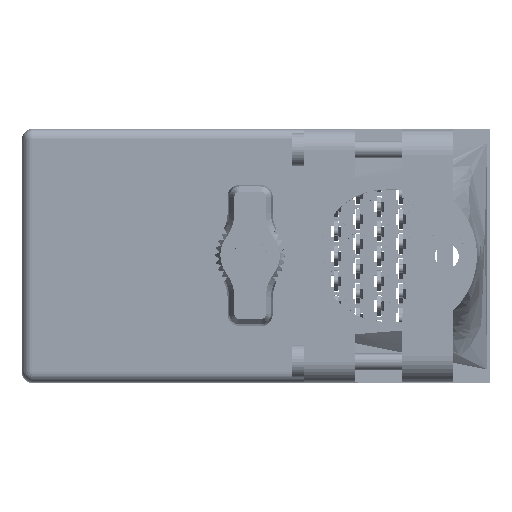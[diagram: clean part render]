
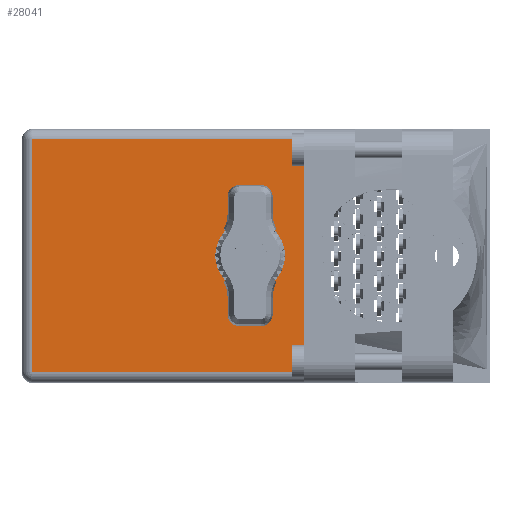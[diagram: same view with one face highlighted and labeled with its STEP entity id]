
A CAD part, top view. The second image highlights one B-rep face of the part: STEP entity #28041.
In plain terms, the highlighted face is planar.
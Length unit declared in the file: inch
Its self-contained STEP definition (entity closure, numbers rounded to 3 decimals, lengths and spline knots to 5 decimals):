
#1946 = DIRECTION ( 'NONE',  ( 1., 0., 0. ) ) ;
#2093 = VERTEX_POINT ( 'NONE', #85353 ) ;
#4004 = CARTESIAN_POINT ( 'NONE',  ( 1.3775, 2.03, -0.765 ) ) ;
#4161 = ORIENTED_EDGE ( 'NONE', *, *, #67292, .T. ) ;
#4527 = AXIS2_PLACEMENT_3D ( 'NONE', #5565, #39660, #73638 ) ;
#4906 = VECTOR ( 'NONE', #41495, 39.37008 ) ;
#5565 = CARTESIAN_POINT ( 'NONE',  ( 0., 2.03, -1.53 ) ) ;
#7499 = CARTESIAN_POINT ( 'NONE',  ( 1.3775, 2.03, -0.6635 ) ) ;
#7896 = CIRCLE ( 'NONE', #96307, 0.1015 ) ;
#8523 = DIRECTION ( 'NONE',  ( -1., 0., 0. ) ) ;
#12904 = VERTEX_POINT ( 'NONE', #34592 ) ;
#14718 = CARTESIAN_POINT ( 'NONE',  ( 1.705, 2.03, -1.468 ) ) ;
#15631 = VECTOR ( 'NONE', #1946, 39.37008 ) ;
#16654 = ORIENTED_EDGE ( 'NONE', *, *, #51481, .F. ) ;
#16913 = LINE ( 'NONE', #26001, #15631 ) ;
#18015 = FACE_OUTER_BOUND ( 'NONE', #84927, .T. ) ;
#18366 = VECTOR ( 'NONE', #41080, 39.37008 ) ;
#19821 = CARTESIAN_POINT ( 'NONE',  ( 1.3775, 2.03, -0.765 ) ) ;
#26001 = CARTESIAN_POINT ( 'NONE',  ( 1.705, 2.03, -0.062 ) ) ;
#28041 = ADVANCED_FACE ( 'NONE', ( #18015, #55131 ), #56711, .T. ) ;
#28339 = DIRECTION ( 'NONE',  ( 0., 0., 1. ) ) ;
#28544 = EDGE_CURVE ( 'NONE', #2093, #86761, #43107, .T. ) ;
#33309 = CARTESIAN_POINT ( 'NONE',  ( 0.062, 2.03, -0.062 ) ) ;
#34592 = CARTESIAN_POINT ( 'NONE',  ( 0.062, 2.03, -1.468 ) ) ;
#36995 = ORIENTED_EDGE ( 'NONE', *, *, #78562, .T. ) ;
#37107 = AXIS2_PLACEMENT_3D ( 'NONE', #4004, #46195, #89056 ) ;
#39353 = VECTOR ( 'NONE', #8523, 39.37008 ) ;
#39660 = DIRECTION ( 'NONE',  ( 0., 1., 0. ) ) ;
#41080 = DIRECTION ( 'NONE',  ( 0., 0., 1. ) ) ;
#41130 = CARTESIAN_POINT ( 'NONE',  ( 1.705, 2.03, -1.53 ) ) ;
#41495 = DIRECTION ( 'NONE',  ( 0., 0., 1. ) ) ;
#43107 = CIRCLE ( 'NONE', #37107, 0.1015 ) ;
#44630 = EDGE_LOOP ( 'NONE', ( #16654, #105317 ) ) ;
#45817 = CARTESIAN_POINT ( 'NONE',  ( 1.705, 2.03, -0.062 ) ) ;
#46195 = DIRECTION ( 'NONE',  ( 0., 1., 0. ) ) ;
#51481 = EDGE_CURVE ( 'NONE', #86761, #2093, #7896, .T. ) ;
#55131 = FACE_BOUND ( 'NONE', #44630, .T. ) ;
#55809 = VERTEX_POINT ( 'NONE', #33309 ) ;
#56711 = PLANE ( 'NONE',  #4527 ) ;
#63601 = ORIENTED_EDGE ( 'NONE', *, *, #83419, .T. ) ;
#65820 = CARTESIAN_POINT ( 'NONE',  ( 0.062, 2.03, -1.53 ) ) ;
#67124 = EDGE_CURVE ( 'NONE', #106046, #87370, #79006, .T. ) ;
#67292 = EDGE_CURVE ( 'NONE', #106046, #12904, #109400, .T. ) ;
#73638 = DIRECTION ( 'NONE',  ( 0., 0., 1. ) ) ;
#77662 = CARTESIAN_POINT ( 'NONE',  ( 0., 2.03, -1.468 ) ) ;
#78562 = EDGE_CURVE ( 'NONE', #55809, #87370, #16913, .T. ) ;
#79006 = LINE ( 'NONE', #41130, #4906 ) ;
#79009 = DIRECTION ( 'NONE',  ( 0., 1., 0. ) ) ;
#83419 = EDGE_CURVE ( 'NONE', #12904, #55809, #91278, .T. ) ;
#84927 = EDGE_LOOP ( 'NONE', ( #63601, #36995, #103962, #4161 ) ) ;
#85353 = CARTESIAN_POINT ( 'NONE',  ( 1.3775, 2.03, -0.8665 ) ) ;
#86761 = VERTEX_POINT ( 'NONE', #7499 ) ;
#87370 = VERTEX_POINT ( 'NONE', #45817 ) ;
#89056 = DIRECTION ( 'NONE',  ( 0., 0., 1. ) ) ;
#91278 = LINE ( 'NONE', #65820, #18366 ) ;
#96307 = AXIS2_PLACEMENT_3D ( 'NONE', #19821, #79009, #28339 ) ;
#103962 = ORIENTED_EDGE ( 'NONE', *, *, #67124, .F. ) ;
#105317 = ORIENTED_EDGE ( 'NONE', *, *, #28544, .F. ) ;
#106046 = VERTEX_POINT ( 'NONE', #14718 ) ;
#109400 = LINE ( 'NONE', #77662, #39353 ) ;
